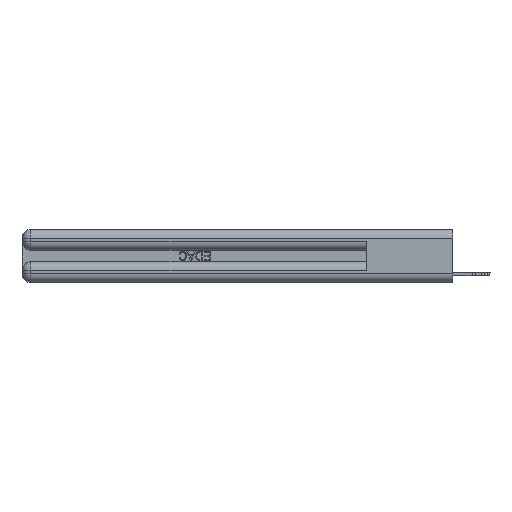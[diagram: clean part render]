
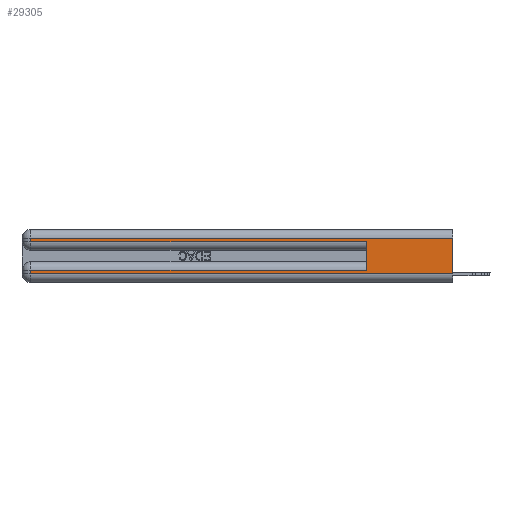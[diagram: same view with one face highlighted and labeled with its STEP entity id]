
A CAD part, left-side view. The second image highlights one B-rep face of the part: STEP entity #29305.
In plain terms, the highlighted planar face has unit normal (-1, 0, 0).
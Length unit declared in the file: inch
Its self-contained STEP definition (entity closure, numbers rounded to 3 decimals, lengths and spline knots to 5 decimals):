
#330 = DIRECTION ( 'NONE',  ( 1., 0., 0. ) ) ;
#341 = CARTESIAN_POINT ( 'NONE',  ( 0., 0., 0.37 ) ) ;
#400 = LINE ( 'NONE', #9830, #29712 ) ;
#793 = VECTOR ( 'NONE', #3245, 39.37008 ) ;
#1045 = ORIENTED_EDGE ( 'NONE', *, *, #11847, .T. ) ;
#1301 = CARTESIAN_POINT ( 'NONE',  ( 0., 0., 0.06 ) ) ;
#1354 = CARTESIAN_POINT ( 'NONE',  ( 0., 0., 0.085 ) ) ;
#1412 = CARTESIAN_POINT ( 'NONE',  ( 0., 0., 0.06 ) ) ;
#1536 = DIRECTION ( 'NONE',  ( 0., 1., 0. ) ) ;
#1663 = EDGE_CURVE ( 'NONE', #5602, #3224, #22117, .T. ) ;
#3224 = VERTEX_POINT ( 'NONE', #1412 ) ;
#3245 = DIRECTION ( 'NONE',  ( 0., 1., 0. ) ) ;
#4087 = VERTEX_POINT ( 'NONE', #28293 ) ;
#5085 = DIRECTION ( 'NONE',  ( 0., 0., 1. ) ) ;
#5602 = VERTEX_POINT ( 'NONE', #8171 ) ;
#5654 = CARTESIAN_POINT ( 'NONE',  ( 0., 0., 0.285 ) ) ;
#5818 = LINE ( 'NONE', #5654, #14624 ) ;
#6759 = CARTESIAN_POINT ( 'NONE',  ( 0., 2.94, 0.06 ) ) ;
#7112 = CARTESIAN_POINT ( 'NONE',  ( 0., 0.6, 0.145 ) ) ;
#8171 = CARTESIAN_POINT ( 'NONE',  ( 0., 0., 0.31 ) ) ;
#8785 = ORIENTED_EDGE ( 'NONE', *, *, #15912, .T. ) ;
#9830 = CARTESIAN_POINT ( 'NONE',  ( 0., 2.94, 0.37 ) ) ;
#9909 = DIRECTION ( 'NONE',  ( 0., 0., -1. ) ) ;
#10437 = EDGE_CURVE ( 'NONE', #25796, #22933, #11874, .T. ) ;
#10475 = LINE ( 'NONE', #1354, #793 ) ;
#11847 = EDGE_CURVE ( 'NONE', #24956, #3224, #25731, .T. ) ;
#11874 = LINE ( 'NONE', #7112, #22490 ) ;
#12831 = ORIENTED_EDGE ( 'NONE', *, *, #27292, .T. ) ;
#12976 = VERTEX_POINT ( 'NONE', #16089 ) ;
#13518 = LINE ( 'NONE', #30375, #25830 ) ;
#14624 = VECTOR ( 'NONE', #20338, 39.37008 ) ;
#14667 = PLANE ( 'NONE',  #24243 ) ;
#15912 = EDGE_CURVE ( 'NONE', #21774, #12976, #27148, .T. ) ;
#16089 = CARTESIAN_POINT ( 'NONE',  ( 0., 2.94, 0.285 ) ) ;
#16646 = CARTESIAN_POINT ( 'NONE',  ( 0., 0.6, 0.085 ) ) ;
#16940 = VECTOR ( 'NONE', #22872, 39.37008 ) ;
#18118 = ORIENTED_EDGE ( 'NONE', *, *, #1663, .F. ) ;
#18350 = DIRECTION ( 'NONE',  ( 0., -1., 0. ) ) ;
#18606 = EDGE_CURVE ( 'NONE', #25796, #4087, #10475, .T. ) ;
#19599 = CARTESIAN_POINT ( 'NONE',  ( 0., 2.94, 0.37 ) ) ;
#19726 = DIRECTION ( 'NONE',  ( 0., 0., -1. ) ) ;
#20338 = DIRECTION ( 'NONE',  ( 0., -1., 0. ) ) ;
#20566 = ORIENTED_EDGE ( 'NONE', *, *, #21468, .T. ) ;
#21468 = EDGE_CURVE ( 'NONE', #5602, #21774, #13518, .T. ) ;
#21774 = VERTEX_POINT ( 'NONE', #27381 ) ;
#21970 = CARTESIAN_POINT ( 'NONE',  ( 0., 0., 0.37 ) ) ;
#22117 = LINE ( 'NONE', #341, #25835 ) ;
#22490 = VECTOR ( 'NONE', #5085, 39.37008 ) ;
#22872 = DIRECTION ( 'NONE',  ( 0., 0., -1. ) ) ;
#22933 = VERTEX_POINT ( 'NONE', #27850 ) ;
#24038 = EDGE_LOOP ( 'NONE', ( #18118, #20566, #8785, #29645, #30069, #24226, #12831, #1045 ) ) ;
#24226 = ORIENTED_EDGE ( 'NONE', *, *, #18606, .T. ) ;
#24243 = AXIS2_PLACEMENT_3D ( 'NONE', #21970, #330, #9909 ) ;
#24956 = VERTEX_POINT ( 'NONE', #6759 ) ;
#25731 = LINE ( 'NONE', #1301, #29436 ) ;
#25796 = VERTEX_POINT ( 'NONE', #16646 ) ;
#25830 = VECTOR ( 'NONE', #1536, 39.37008 ) ;
#25835 = VECTOR ( 'NONE', #19726, 39.37008 ) ;
#27148 = LINE ( 'NONE', #19599, #16940 ) ;
#27292 = EDGE_CURVE ( 'NONE', #4087, #24956, #400, .T. ) ;
#27381 = CARTESIAN_POINT ( 'NONE',  ( 0., 2.94, 0.31 ) ) ;
#27850 = CARTESIAN_POINT ( 'NONE',  ( 0., 0.6, 0.285 ) ) ;
#28260 = EDGE_CURVE ( 'NONE', #12976, #22933, #5818, .T. ) ;
#28293 = CARTESIAN_POINT ( 'NONE',  ( 0., 2.94, 0.085 ) ) ;
#29015 = FACE_OUTER_BOUND ( 'NONE', #24038, .T. ) ;
#29305 = ADVANCED_FACE ( 'NONE', ( #29015 ), #14667, .F. ) ;
#29436 = VECTOR ( 'NONE', #18350, 39.37008 ) ;
#29546 = DIRECTION ( 'NONE',  ( 0., 0., -1. ) ) ;
#29645 = ORIENTED_EDGE ( 'NONE', *, *, #28260, .T. ) ;
#29712 = VECTOR ( 'NONE', #29546, 39.37008 ) ;
#30069 = ORIENTED_EDGE ( 'NONE', *, *, #10437, .F. ) ;
#30375 = CARTESIAN_POINT ( 'NONE',  ( 0., 0., 0.31 ) ) ;
